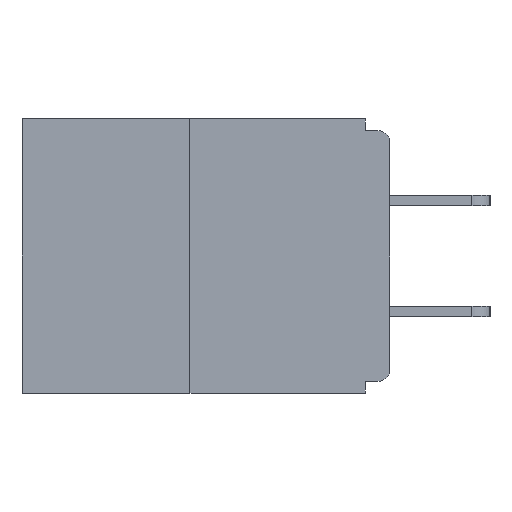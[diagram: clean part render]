
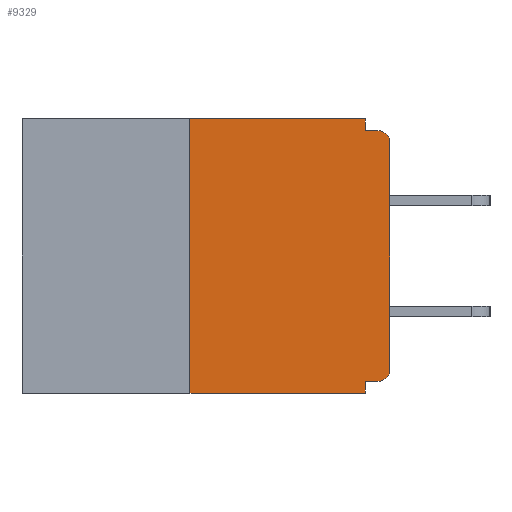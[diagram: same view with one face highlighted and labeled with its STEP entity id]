
A CAD part, left-side view. The second image highlights one B-rep face of the part: STEP entity #9329.
In plain terms, the highlighted planar face has unit normal (-1, 0, 0).
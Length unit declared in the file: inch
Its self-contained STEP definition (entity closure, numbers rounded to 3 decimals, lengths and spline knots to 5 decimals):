
#186 = VERTEX_POINT ( 'NONE', #11809 ) ;
#434 = CARTESIAN_POINT ( 'NONE',  ( 0., 0., -0.015 ) ) ;
#466 = VERTEX_POINT ( 'NONE', #9745 ) ;
#609 = DIRECTION ( 'NONE',  ( 0., -1., 0. ) ) ;
#685 = PLANE ( 'NONE',  #2386 ) ;
#745 = FACE_OUTER_BOUND ( 'NONE', #11713, .T. ) ;
#852 = CARTESIAN_POINT ( 'NONE',  ( 0., 0.46, -0.343 ) ) ;
#995 = CIRCLE ( 'NONE', #7898, 0.015 ) ;
#1174 = CARTESIAN_POINT ( 'NONE',  ( 0., 0.031, -0.015 ) ) ;
#1190 = EDGE_CURVE ( 'NONE', #5732, #186, #2135, .T. ) ;
#1374 = CARTESIAN_POINT ( 'NONE',  ( 0., 0.25, 0. ) ) ;
#1447 = CARTESIAN_POINT ( 'NONE',  ( 0., 0.031, -0.343 ) ) ;
#1546 = DIRECTION ( 'NONE',  ( 0., 0., -1. ) ) ;
#1610 = VERTEX_POINT ( 'NONE', #11601 ) ;
#1737 = EDGE_CURVE ( 'NONE', #466, #5732, #2100, .T. ) ;
#2100 = LINE ( 'NONE', #10799, #5512 ) ;
#2135 = CIRCLE ( 'NONE', #4921, 0.015 ) ;
#2351 = DIRECTION ( 'NONE',  ( 0., 0., 1. ) ) ;
#2386 = AXIS2_PLACEMENT_3D ( 'NONE', #5382, #3384, #4592 ) ;
#2548 = CARTESIAN_POINT ( 'NONE',  ( 0., 0.031, 0. ) ) ;
#2648 = CARTESIAN_POINT ( 'NONE',  ( 0., 0.031, 0. ) ) ;
#2992 = CARTESIAN_POINT ( 'NONE',  ( 0., 0.25, 0. ) ) ;
#3209 = ORIENTED_EDGE ( 'NONE', *, *, #6680, .F. ) ;
#3384 = DIRECTION ( 'NONE',  ( 1., 0., 0. ) ) ;
#3510 = EDGE_CURVE ( 'NONE', #5168, #466, #995, .T. ) ;
#3637 = DIRECTION ( 'NONE',  ( 0., 0., -1. ) ) ;
#3680 = VECTOR ( 'NONE', #4338, 39.37008 ) ;
#3685 = DIRECTION ( 'NONE',  ( -1., 0., 0. ) ) ;
#3774 = ORIENTED_EDGE ( 'NONE', *, *, #10852, .F. ) ;
#3860 = VERTEX_POINT ( 'NONE', #5122 ) ;
#4088 = CARTESIAN_POINT ( 'NONE',  ( 0., 0.015, -0.328 ) ) ;
#4305 = DIRECTION ( 'NONE',  ( 0., 0., -1. ) ) ;
#4338 = DIRECTION ( 'NONE',  ( 0., -1., 0. ) ) ;
#4592 = DIRECTION ( 'NONE',  ( 0., 0., -1. ) ) ;
#4666 = LINE ( 'NONE', #1447, #10566 ) ;
#4739 = CARTESIAN_POINT ( 'NONE',  ( 0., 0.015, -0.313 ) ) ;
#4896 = VECTOR ( 'NONE', #7611, 39.37008 ) ;
#4921 = AXIS2_PLACEMENT_3D ( 'NONE', #10157, #12056, #3637 ) ;
#5122 = CARTESIAN_POINT ( 'NONE',  ( 0., 0.031, -0.328 ) ) ;
#5168 = VERTEX_POINT ( 'NONE', #4088 ) ;
#5382 = CARTESIAN_POINT ( 'NONE',  ( 0., 0.46, 0. ) ) ;
#5487 = VECTOR ( 'NONE', #1546, 39.37008 ) ;
#5498 = LINE ( 'NONE', #5729, #4896 ) ;
#5512 = VECTOR ( 'NONE', #2351, 39.37008 ) ;
#5729 = CARTESIAN_POINT ( 'NONE',  ( 0., 0.46, 0. ) ) ;
#5732 = VERTEX_POINT ( 'NONE', #9460 ) ;
#5828 = ORIENTED_EDGE ( 'NONE', *, *, #1190, .T. ) ;
#6104 = ORIENTED_EDGE ( 'NONE', *, *, #1737, .T. ) ;
#6680 = EDGE_CURVE ( 'NONE', #7889, #186, #7189, .T. ) ;
#6991 = ORIENTED_EDGE ( 'NONE', *, *, #10028, .F. ) ;
#7189 = LINE ( 'NONE', #434, #3680 ) ;
#7209 = LINE ( 'NONE', #1374, #11271 ) ;
#7413 = DIRECTION ( 'NONE',  ( 0., 0., -1. ) ) ;
#7611 = DIRECTION ( 'NONE',  ( 0., -1., 0. ) ) ;
#7889 = VERTEX_POINT ( 'NONE', #1174 ) ;
#7898 = AXIS2_PLACEMENT_3D ( 'NONE', #4739, #3685, #7413 ) ;
#7910 = LINE ( 'NONE', #11643, #8121 ) ;
#8024 = EDGE_CURVE ( 'NONE', #10808, #7889, #8076, .T. ) ;
#8049 = VERTEX_POINT ( 'NONE', #9182 ) ;
#8076 = LINE ( 'NONE', #2648, #5487 ) ;
#8121 = VECTOR ( 'NONE', #10109, 39.37008 ) ;
#8296 = VERTEX_POINT ( 'NONE', #2992 ) ;
#8325 = LINE ( 'NONE', #852, #8914 ) ;
#8614 = EDGE_CURVE ( 'NONE', #8296, #10808, #5498, .T. ) ;
#8810 = ORIENTED_EDGE ( 'NONE', *, *, #8614, .F. ) ;
#8837 = EDGE_CURVE ( 'NONE', #3860, #8049, #4666, .T. ) ;
#8849 = ORIENTED_EDGE ( 'NONE', *, *, #10518, .T. ) ;
#8914 = VECTOR ( 'NONE', #609, 39.37008 ) ;
#9182 = CARTESIAN_POINT ( 'NONE',  ( 0., 0.031, -0.343 ) ) ;
#9329 = ADVANCED_FACE ( 'NONE', ( #745 ), #685, .F. ) ;
#9460 = CARTESIAN_POINT ( 'NONE',  ( 0., 0., -0.03 ) ) ;
#9503 = ORIENTED_EDGE ( 'NONE', *, *, #8837, .F. ) ;
#9745 = CARTESIAN_POINT ( 'NONE',  ( 0., 0., -0.313 ) ) ;
#10028 = EDGE_CURVE ( 'NONE', #5168, #3860, #7910, .T. ) ;
#10109 = DIRECTION ( 'NONE',  ( 0., 1., 0. ) ) ;
#10157 = CARTESIAN_POINT ( 'NONE',  ( 0., 0.015, -0.03 ) ) ;
#10518 = EDGE_CURVE ( 'NONE', #1610, #8049, #8325, .T. ) ;
#10566 = VECTOR ( 'NONE', #4305, 39.37008 ) ;
#10799 = CARTESIAN_POINT ( 'NONE',  ( 0., 0., 0. ) ) ;
#10805 = DIRECTION ( 'NONE',  ( 0., 0., 1. ) ) ;
#10808 = VERTEX_POINT ( 'NONE', #2548 ) ;
#10852 = EDGE_CURVE ( 'NONE', #1610, #8296, #7209, .T. ) ;
#11271 = VECTOR ( 'NONE', #10805, 39.37008 ) ;
#11601 = CARTESIAN_POINT ( 'NONE',  ( 0., 0.25, -0.343 ) ) ;
#11643 = CARTESIAN_POINT ( 'NONE',  ( 0., 0., -0.328 ) ) ;
#11713 = EDGE_LOOP ( 'NONE', ( #8810, #3774, #8849, #9503, #6991, #11803, #6104, #5828, #3209, #12008 ) ) ;
#11803 = ORIENTED_EDGE ( 'NONE', *, *, #3510, .T. ) ;
#11809 = CARTESIAN_POINT ( 'NONE',  ( 0., 0.015, -0.015 ) ) ;
#12008 = ORIENTED_EDGE ( 'NONE', *, *, #8024, .F. ) ;
#12056 = DIRECTION ( 'NONE',  ( -1., 0., 0. ) ) ;
